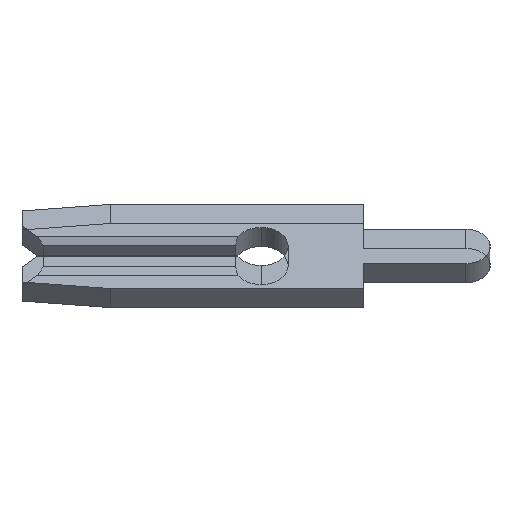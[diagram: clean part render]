
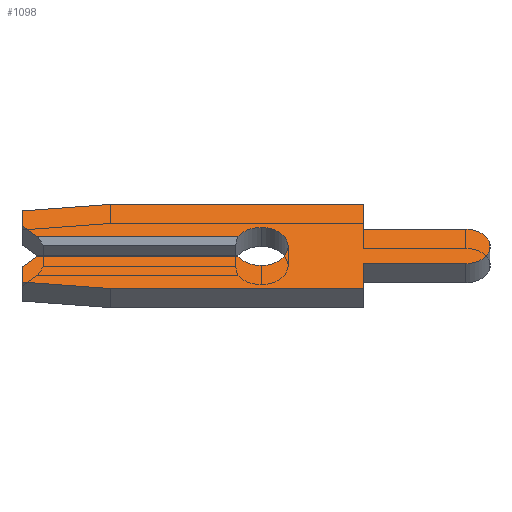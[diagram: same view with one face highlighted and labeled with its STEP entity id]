
A CAD part, left-side view. The second image highlights one B-rep face of the part: STEP entity #1098.
In plain terms, the highlighted face is planar.
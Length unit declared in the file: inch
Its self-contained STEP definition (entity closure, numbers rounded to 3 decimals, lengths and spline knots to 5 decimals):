
#3 = CARTESIAN_POINT ( 'NONE',  ( -0.013, 0., 0. ) ) ;
#18 = EDGE_CURVE ( 'NONE', #1614, #505, #1549, .T. ) ;
#44 = ORIENTED_EDGE ( 'NONE', *, *, #1301, .F. ) ;
#53 = CARTESIAN_POINT ( 'NONE',  ( -0.013, 0.231, 0.013 ) ) ;
#54 = AXIS2_PLACEMENT_3D ( 'NONE', #1908, #1969, #2002 ) ;
#63 = VECTOR ( 'NONE', #920, 39.37008 ) ;
#66 = CARTESIAN_POINT ( 'NONE',  ( -0.013, 0., -0.026 ) ) ;
#90 = ORIENTED_EDGE ( 'NONE', *, *, #1013, .F. ) ;
#127 = VECTOR ( 'NONE', #1273, 39.37008 ) ;
#154 = PLANE ( 'NONE',  #1030 ) ;
#182 = VERTEX_POINT ( 'NONE', #905 ) ;
#215 = LINE ( 'NONE', #1698, #2612 ) ;
#316 = LINE ( 'NONE', #1103, #1943 ) ;
#324 = VERTEX_POINT ( 'NONE', #66 ) ;
#329 = CARTESIAN_POINT ( 'NONE',  ( -0.013, 0.02252, 0.013 ) ) ;
#347 = ORIENTED_EDGE ( 'NONE', *, *, #1123, .F. ) ;
#348 = DIRECTION ( 'NONE',  ( 0., 0.995, 0.105 ) ) ;
#376 = DIRECTION ( 'NONE',  ( 0., 1., 0. ) ) ;
#379 = VERTEX_POINT ( 'NONE', #2263 ) ;
#387 = LINE ( 'NONE', #536, #2026 ) ;
#428 = CARTESIAN_POINT ( 'NONE',  ( -0.013, 0., 0. ) ) ;
#447 = CARTESIAN_POINT ( 'NONE',  ( -0.013, -0.099, -0.0235 ) ) ;
#455 = EDGE_LOOP ( 'NONE', ( #1548, #875, #1071, #1306, #777, #90, #44, #2090, #528, #1012, #1066, #1701, #2315, #1713, #1815, #347, #1011, #909 ) ) ;
#505 = VERTEX_POINT ( 'NONE', #951 ) ;
#526 = CARTESIAN_POINT ( 'NONE',  ( -0.013, 0.231, 0.028 ) ) ;
#528 = ORIENTED_EDGE ( 'NONE', *, *, #2155, .F. ) ;
#536 = CARTESIAN_POINT ( 'NONE',  ( -0.013, 0., -0.013 ) ) ;
#555 = VERTEX_POINT ( 'NONE', #932 ) ;
#603 = LINE ( 'NONE', #2544, #944 ) ;
#654 = VECTOR ( 'NONE', #2375, 39.37008 ) ;
#664 = VERTEX_POINT ( 'NONE', #1398 ) ;
#733 = FACE_OUTER_BOUND ( 'NONE', #455, .T. ) ;
#777 = ORIENTED_EDGE ( 'NONE', *, *, #788, .F. ) ;
#788 = EDGE_CURVE ( 'NONE', #2527, #874, #387, .T. ) ;
#793 = CARTESIAN_POINT ( 'NONE',  ( -0.013, 0.231, -0.04857 ) ) ;
#805 = LINE ( 'NONE', #1486, #2526 ) ;
#874 = VERTEX_POINT ( 'NONE', #2290 ) ;
#875 = ORIENTED_EDGE ( 'NONE', *, *, #1567, .F. ) ;
#883 = EDGE_CURVE ( 'NONE', #664, #1046, #1848, .T. ) ;
#905 = CARTESIAN_POINT ( 'NONE',  ( -0.013, -0.099, 0.0575 ) ) ;
#909 = ORIENTED_EDGE ( 'NONE', *, *, #883, .F. ) ;
#914 = VERTEX_POINT ( 'NONE', #329 ) ;
#920 = DIRECTION ( 'NONE',  ( 0., -1., 0. ) ) ;
#932 = CARTESIAN_POINT ( 'NONE',  ( -0.013, 0., 0.026 ) ) ;
#943 = CIRCLE ( 'NONE', #54, 0.0235 ) ;
#944 = VECTOR ( 'NONE', #1870, 39.37008 ) ;
#951 = CARTESIAN_POINT ( 'NONE',  ( -0.013, -0.099, -0.0575 ) ) ;
#979 = CARTESIAN_POINT ( 'NONE',  ( -0.013, 0.2105, -0.0075 ) ) ;
#1005 = LINE ( 'NONE', #1734, #127 ) ;
#1011 = ORIENTED_EDGE ( 'NONE', *, *, #1553, .F. ) ;
#1012 = ORIENTED_EDGE ( 'NONE', *, *, #18, .F. ) ;
#1013 = EDGE_CURVE ( 'NONE', #1784, #2527, #2272, .T. ) ;
#1030 = AXIS2_PLACEMENT_3D ( 'NONE', #1470, #2043, #1282 ) ;
#1046 = VERTEX_POINT ( 'NONE', #526 ) ;
#1066 = ORIENTED_EDGE ( 'NONE', *, *, #1363, .F. ) ;
#1071 = ORIENTED_EDGE ( 'NONE', *, *, #1422, .F. ) ;
#1098 = ADVANCED_FACE ( 'NONE', ( #733 ), #154, .F. ) ;
#1103 = CARTESIAN_POINT ( 'NONE',  ( -0.013, 0.146, -0.0575 ) ) ;
#1123 = EDGE_CURVE ( 'NONE', #379, #1441, #603, .T. ) ;
#1179 = LINE ( 'NONE', #1772, #2524 ) ;
#1273 = DIRECTION ( 'NONE',  ( 0., 0., -1. ) ) ;
#1282 = DIRECTION ( 'NONE',  ( 0., 0., -1. ) ) ;
#1301 = EDGE_CURVE ( 'NONE', #1380, #1784, #2683, .T. ) ;
#1306 = ORIENTED_EDGE ( 'NONE', *, *, #1924, .F. ) ;
#1309 = LINE ( 'NONE', #2172, #2640 ) ;
#1316 = VERTEX_POINT ( 'NONE', #2559 ) ;
#1342 = VECTOR ( 'NONE', #2299, 39.37008 ) ;
#1363 = EDGE_CURVE ( 'NONE', #1679, #1614, #805, .T. ) ;
#1380 = VERTEX_POINT ( 'NONE', #793 ) ;
#1398 = CARTESIAN_POINT ( 'NONE',  ( -0.013, 0.216, 0.013 ) ) ;
#1411 = EDGE_CURVE ( 'NONE', #1316, #1380, #215, .T. ) ;
#1422 = EDGE_CURVE ( 'NONE', #324, #555, #1620, .T. ) ;
#1441 = VERTEX_POINT ( 'NONE', #1677 ) ;
#1470 = CARTESIAN_POINT ( 'NONE',  ( -0.013, 0., 0. ) ) ;
#1486 = CARTESIAN_POINT ( 'NONE',  ( -0.013, -0.099, -0.0235 ) ) ;
#1514 = DIRECTION ( 'NONE',  ( 0., 0., -1. ) ) ;
#1546 = LINE ( 'NONE', #53, #63 ) ;
#1547 = VERTEX_POINT ( 'NONE', #2585 ) ;
#1548 = ORIENTED_EDGE ( 'NONE', *, *, #1904, .T. ) ;
#1549 = LINE ( 'NONE', #1788, #2399 ) ;
#1553 = EDGE_CURVE ( 'NONE', #1046, #379, #1309, .T. ) ;
#1565 = CARTESIAN_POINT ( 'NONE',  ( -0.013, 0., 0. ) ) ;
#1567 = EDGE_CURVE ( 'NONE', #555, #914, #2333, .T. ) ;
#1591 = EDGE_CURVE ( 'NONE', #1441, #182, #2224, .T. ) ;
#1598 = DIRECTION ( 'NONE',  ( -1., 0., 0. ) ) ;
#1614 = VERTEX_POINT ( 'NONE', #447 ) ;
#1620 = CIRCLE ( 'NONE', #2301, 0.026 ) ;
#1630 = DIRECTION ( 'NONE',  ( 0., -1., 0. ) ) ;
#1659 = AXIS2_PLACEMENT_3D ( 'NONE', #428, #1915, #1514 ) ;
#1677 = CARTESIAN_POINT ( 'NONE',  ( -0.013, 0.146, 0.0575 ) ) ;
#1679 = VERTEX_POINT ( 'NONE', #1939 ) ;
#1698 = CARTESIAN_POINT ( 'NONE',  ( -0.013, 0.231, -0.04857 ) ) ;
#1701 = ORIENTED_EDGE ( 'NONE', *, *, #1738, .F. ) ;
#1706 = DIRECTION ( 'NONE',  ( 0., 0., -1. ) ) ;
#1709 = DIRECTION ( 'NONE',  ( 0., 1., 0. ) ) ;
#1713 = ORIENTED_EDGE ( 'NONE', *, *, #2209, .F. ) ;
#1729 = CARTESIAN_POINT ( 'NONE',  ( -0.013, 0.146, 0.0575 ) ) ;
#1734 = CARTESIAN_POINT ( 'NONE',  ( -0.013, -0.099, 0.0575 ) ) ;
#1738 = EDGE_CURVE ( 'NONE', #1547, #1679, #943, .T. ) ;
#1772 = CARTESIAN_POINT ( 'NONE',  ( -0.013, -0.099, 0.0235 ) ) ;
#1784 = VERTEX_POINT ( 'NONE', #1990 ) ;
#1788 = CARTESIAN_POINT ( 'NONE',  ( -0.013, -0.099, -0.0575 ) ) ;
#1815 = ORIENTED_EDGE ( 'NONE', *, *, #1591, .F. ) ;
#1820 = VECTOR ( 'NONE', #2349, 39.37008 ) ;
#1827 = DIRECTION ( 'NONE',  ( 0., -0.707, 0.707 ) ) ;
#1848 = LINE ( 'NONE', #2079, #1342 ) ;
#1870 = DIRECTION ( 'NONE',  ( 0., -0.995, 0.105 ) ) ;
#1904 = EDGE_CURVE ( 'NONE', #664, #914, #1546, .T. ) ;
#1908 = CARTESIAN_POINT ( 'NONE',  ( -0.013, -0.1975, 0. ) ) ;
#1911 = VECTOR ( 'NONE', #1827, 39.37008 ) ;
#1915 = DIRECTION ( 'NONE',  ( -1., 0., 0. ) ) ;
#1924 = EDGE_CURVE ( 'NONE', #874, #324, #2583, .T. ) ;
#1939 = CARTESIAN_POINT ( 'NONE',  ( -0.013, -0.1975, -0.0235 ) ) ;
#1943 = VECTOR ( 'NONE', #1709, 39.37008 ) ;
#1969 = DIRECTION ( 'NONE',  ( 1., 0., 0. ) ) ;
#1973 = CARTESIAN_POINT ( 'NONE',  ( -0.013, 0.216, -0.013 ) ) ;
#1990 = CARTESIAN_POINT ( 'NONE',  ( -0.013, 0.231, -0.028 ) ) ;
#2002 = DIRECTION ( 'NONE',  ( 0., 0., 1. ) ) ;
#2026 = VECTOR ( 'NONE', #1630, 39.37008 ) ;
#2035 = DIRECTION ( 'NONE',  ( 0., 0., -1. ) ) ;
#2043 = DIRECTION ( 'NONE',  ( 1., 0., 0. ) ) ;
#2079 = CARTESIAN_POINT ( 'NONE',  ( -0.013, 0.2105, 0.0075 ) ) ;
#2090 = ORIENTED_EDGE ( 'NONE', *, *, #1411, .F. ) ;
#2155 = EDGE_CURVE ( 'NONE', #505, #1316, #316, .T. ) ;
#2172 = CARTESIAN_POINT ( 'NONE',  ( -0.013, 0.231, 0.028 ) ) ;
#2186 = DIRECTION ( 'NONE',  ( -1., 0., 0. ) ) ;
#2209 = EDGE_CURVE ( 'NONE', #182, #2651, #1005, .T. ) ;
#2224 = LINE ( 'NONE', #1729, #654 ) ;
#2263 = CARTESIAN_POINT ( 'NONE',  ( -0.013, 0.231, 0.04857 ) ) ;
#2272 = LINE ( 'NONE', #979, #1911 ) ;
#2290 = CARTESIAN_POINT ( 'NONE',  ( -0.013, 0.02252, -0.013 ) ) ;
#2299 = DIRECTION ( 'NONE',  ( 0., 0.707, 0.707 ) ) ;
#2301 = AXIS2_PLACEMENT_3D ( 'NONE', #3, #2186, #1706 ) ;
#2315 = ORIENTED_EDGE ( 'NONE', *, *, #2437, .F. ) ;
#2318 = CARTESIAN_POINT ( 'NONE',  ( -0.013, 0.231, -0.028 ) ) ;
#2333 = CIRCLE ( 'NONE', #1659, 0.026 ) ;
#2349 = DIRECTION ( 'NONE',  ( 0., 0., 1. ) ) ;
#2375 = DIRECTION ( 'NONE',  ( 0., -1., 0. ) ) ;
#2399 = VECTOR ( 'NONE', #2465, 39.37008 ) ;
#2415 = CARTESIAN_POINT ( 'NONE',  ( -0.013, -0.099, 0.0235 ) ) ;
#2437 = EDGE_CURVE ( 'NONE', #2651, #1547, #1179, .T. ) ;
#2465 = DIRECTION ( 'NONE',  ( 0., 0., -1. ) ) ;
#2524 = VECTOR ( 'NONE', #2617, 39.37008 ) ;
#2526 = VECTOR ( 'NONE', #376, 39.37008 ) ;
#2527 = VERTEX_POINT ( 'NONE', #1973 ) ;
#2544 = CARTESIAN_POINT ( 'NONE',  ( -0.013, 0.231, 0.04857 ) ) ;
#2559 = CARTESIAN_POINT ( 'NONE',  ( -0.013, 0.146, -0.0575 ) ) ;
#2583 = CIRCLE ( 'NONE', #2698, 0.026 ) ;
#2585 = CARTESIAN_POINT ( 'NONE',  ( -0.013, -0.1975, 0.0235 ) ) ;
#2594 = DIRECTION ( 'NONE',  ( 0., 0., 1. ) ) ;
#2612 = VECTOR ( 'NONE', #348, 39.37008 ) ;
#2617 = DIRECTION ( 'NONE',  ( 0., -1., 0. ) ) ;
#2640 = VECTOR ( 'NONE', #2594, 39.37008 ) ;
#2651 = VERTEX_POINT ( 'NONE', #2415 ) ;
#2683 = LINE ( 'NONE', #2318, #1820 ) ;
#2698 = AXIS2_PLACEMENT_3D ( 'NONE', #1565, #1598, #2035 ) ;
